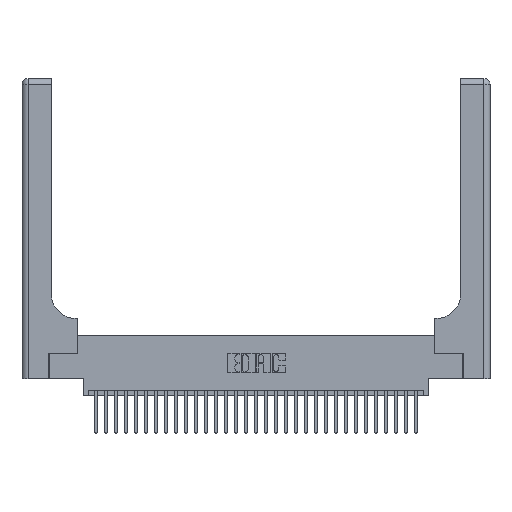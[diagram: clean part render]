
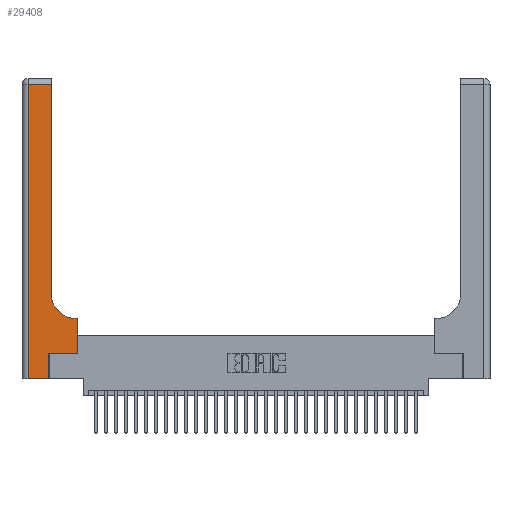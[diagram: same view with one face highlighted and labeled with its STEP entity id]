
A CAD part, top view. The second image highlights one B-rep face of the part: STEP entity #29408.
In plain terms, the highlighted planar face has unit normal (0, 0, 1).
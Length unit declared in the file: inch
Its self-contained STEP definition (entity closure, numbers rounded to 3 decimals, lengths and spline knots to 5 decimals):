
#239 = ORIENTED_EDGE ( 'NONE', *, *, #23862, .T. ) ;
#779 = EDGE_CURVE ( 'NONE', #8605, #29764, #26382, .T. ) ;
#839 = DIRECTION ( 'NONE',  ( -1., 0., 0. ) ) ;
#2724 = EDGE_CURVE ( 'NONE', #16823, #3266, #9330, .T. ) ;
#2783 = DIRECTION ( 'NONE',  ( 0., 0., -1. ) ) ;
#3108 = CARTESIAN_POINT ( 'NONE',  ( 0., 2.94, 0.37 ) ) ;
#3142 = CARTESIAN_POINT ( 'NONE',  ( 0.5585, 0.6, 0.37 ) ) ;
#3215 = EDGE_CURVE ( 'NONE', #28548, #15153, #18309, .T. ) ;
#3266 = VERTEX_POINT ( 'NONE', #19123 ) ;
#3357 = ORIENTED_EDGE ( 'NONE', *, *, #3215, .T. ) ;
#4410 = VECTOR ( 'NONE', #31354, 39.37008 ) ;
#4602 = DIRECTION ( 'NONE',  ( 1., 0., 0. ) ) ;
#4776 = VECTOR ( 'NONE', #15059, 39.37008 ) ;
#6370 = LINE ( 'NONE', #30592, #4776 ) ;
#7162 = ORIENTED_EDGE ( 'NONE', *, *, #19851, .T. ) ;
#7454 = CARTESIAN_POINT ( 'NONE',  ( 0.269, 0., 0.37 ) ) ;
#8236 = CARTESIAN_POINT ( 'NONE',  ( 0.2915, 0.6, 0.37 ) ) ;
#8455 = DIRECTION ( 'NONE',  ( 1., 0., 0. ) ) ;
#8605 = VERTEX_POINT ( 'NONE', #15566 ) ;
#8881 = CARTESIAN_POINT ( 'NONE',  ( 0.269, 0.25, 0.37 ) ) ;
#8888 = DIRECTION ( 'NONE',  ( 0., 1., 0. ) ) ;
#9330 = LINE ( 'NONE', #8236, #23110 ) ;
#9712 = LINE ( 'NONE', #3108, #26605 ) ;
#10699 = DIRECTION ( 'NONE',  ( -1., 0., 0. ) ) ;
#11043 = DIRECTION ( 'NONE',  ( 0., 0., -1. ) ) ;
#11469 = VERTEX_POINT ( 'NONE', #24358 ) ;
#12533 = FACE_OUTER_BOUND ( 'NONE', #17377, .T. ) ;
#12842 = CARTESIAN_POINT ( 'NONE',  ( 0.2915, 2.94, 0.37 ) ) ;
#14044 = CIRCLE ( 'NONE', #31955, 0.25 ) ;
#15059 = DIRECTION ( 'NONE',  ( 0., 1., 0. ) ) ;
#15105 = VECTOR ( 'NONE', #8455, 39.37008 ) ;
#15120 = CARTESIAN_POINT ( 'NONE',  ( 0.06, 0., 0.37 ) ) ;
#15153 = VERTEX_POINT ( 'NONE', #18521 ) ;
#15164 = VECTOR ( 'NONE', #4602, 39.37008 ) ;
#15272 = CARTESIAN_POINT ( 'NONE',  ( 0.2915, 3., 0.37 ) ) ;
#15422 = VECTOR ( 'NONE', #23176, 39.37008 ) ;
#15566 = CARTESIAN_POINT ( 'NONE',  ( 0.06, 2.94, 0.37 ) ) ;
#16823 = VERTEX_POINT ( 'NONE', #3142 ) ;
#17377 = EDGE_LOOP ( 'NONE', ( #7162, #26537, #23435, #23822, #3357, #18961, #19218, #24302, #239 ) ) ;
#17568 = AXIS2_PLACEMENT_3D ( 'NONE', #21388, #11043, #26322 ) ;
#18228 = CARTESIAN_POINT ( 'NONE',  ( 0.5415, 0.85, 0.37 ) ) ;
#18249 = EDGE_CURVE ( 'NONE', #29764, #28548, #22634, .T. ) ;
#18309 = LINE ( 'NONE', #19814, #26599 ) ;
#18521 = CARTESIAN_POINT ( 'NONE',  ( 0.269, 0.25, 0.37 ) ) ;
#18961 = ORIENTED_EDGE ( 'NONE', *, *, #26554, .T. ) ;
#19123 = CARTESIAN_POINT ( 'NONE',  ( 0.5415, 0.6, 0.37 ) ) ;
#19218 = ORIENTED_EDGE ( 'NONE', *, *, #20727, .T. ) ;
#19487 = CARTESIAN_POINT ( 'NONE',  ( 0., 0., 0.37 ) ) ;
#19804 = VERTEX_POINT ( 'NONE', #12842 ) ;
#19814 = CARTESIAN_POINT ( 'NONE',  ( 0.269, 0., 0.37 ) ) ;
#19851 = EDGE_CURVE ( 'NONE', #31677, #19804, #22095, .T. ) ;
#20727 = EDGE_CURVE ( 'NONE', #11469, #16823, #6370, .T. ) ;
#21161 = PLANE ( 'NONE',  #17568 ) ;
#21388 = CARTESIAN_POINT ( 'NONE',  ( 0., 3., 0.37 ) ) ;
#22095 = LINE ( 'NONE', #15272, #15422 ) ;
#22566 = LINE ( 'NONE', #8881, #15105 ) ;
#22634 = LINE ( 'NONE', #19487, #15164 ) ;
#23110 = VECTOR ( 'NONE', #839, 39.37008 ) ;
#23176 = DIRECTION ( 'NONE',  ( 0., 1., 0. ) ) ;
#23435 = ORIENTED_EDGE ( 'NONE', *, *, #779, .T. ) ;
#23798 = EDGE_CURVE ( 'NONE', #19804, #8605, #9712, .T. ) ;
#23822 = ORIENTED_EDGE ( 'NONE', *, *, #18249, .T. ) ;
#23862 = EDGE_CURVE ( 'NONE', #3266, #31677, #14044, .T. ) ;
#24302 = ORIENTED_EDGE ( 'NONE', *, *, #2724, .T. ) ;
#24358 = CARTESIAN_POINT ( 'NONE',  ( 0.5585, 0.25, 0.37 ) ) ;
#25552 = CARTESIAN_POINT ( 'NONE',  ( 0.2915, 0.85, 0.37 ) ) ;
#26322 = DIRECTION ( 'NONE',  ( -1., 0., 0. ) ) ;
#26382 = LINE ( 'NONE', #29393, #4410 ) ;
#26537 = ORIENTED_EDGE ( 'NONE', *, *, #23798, .T. ) ;
#26554 = EDGE_CURVE ( 'NONE', #15153, #11469, #22566, .T. ) ;
#26599 = VECTOR ( 'NONE', #8888, 39.37008 ) ;
#26605 = VECTOR ( 'NONE', #10699, 39.37008 ) ;
#28034 = DIRECTION ( 'NONE',  ( 1., 0., 0. ) ) ;
#28548 = VERTEX_POINT ( 'NONE', #7454 ) ;
#29393 = CARTESIAN_POINT ( 'NONE',  ( 0.06, 3., 0.37 ) ) ;
#29408 = ADVANCED_FACE ( 'NONE', ( #12533 ), #21161, .F. ) ;
#29764 = VERTEX_POINT ( 'NONE', #15120 ) ;
#30592 = CARTESIAN_POINT ( 'NONE',  ( 0.5585, 0.25, 0.37 ) ) ;
#31354 = DIRECTION ( 'NONE',  ( 0., -1., 0. ) ) ;
#31677 = VERTEX_POINT ( 'NONE', #25552 ) ;
#31955 = AXIS2_PLACEMENT_3D ( 'NONE', #18228, #2783, #28034 ) ;
